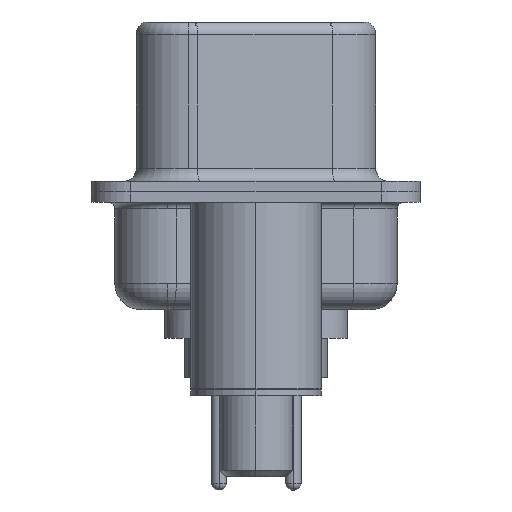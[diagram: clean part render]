
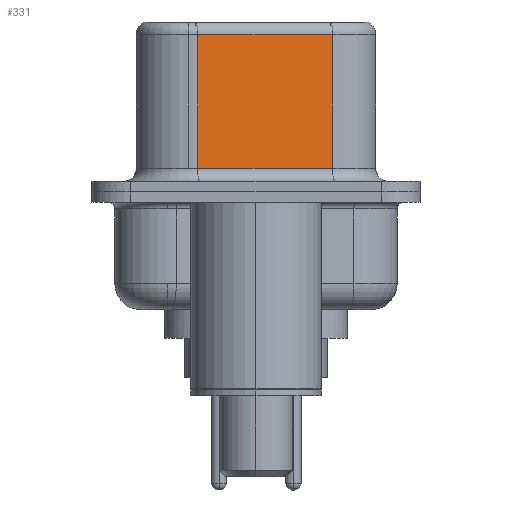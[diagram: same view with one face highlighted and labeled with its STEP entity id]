
A CAD part, left-side view. The second image highlights one B-rep face of the part: STEP entity #331.
In plain terms, the highlighted planar face has unit normal (-0.985, -0.174, 0).
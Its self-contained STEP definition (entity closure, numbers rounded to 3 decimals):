
#331 = ADVANCED_FACE ( 'NONE', ( #4750 ), #9313, .F. ) ;
#768 = ORIENTED_EDGE ( 'NONE', *, *, #12194, .T. ) ;
#1760 = DIRECTION ( 'NONE',  ( 0.174, -0.985, 0. ) ) ;
#2746 = CARTESIAN_POINT ( 'NONE',  ( 3.67, 2.233, 6.52 ) ) ;
#3579 = LINE ( 'NONE', #2746, #11378 ) ;
#4750 = FACE_OUTER_BOUND ( 'NONE', #9979, .T. ) ;
#4772 = ORIENTED_EDGE ( 'NONE', *, *, #19512, .T. ) ;
#5371 = VECTOR ( 'NONE', #1760, 1000. ) ;
#5804 = ORIENTED_EDGE ( 'NONE', *, *, #12025, .F. ) ;
#6564 = VECTOR ( 'NONE', #10188, 1000. ) ;
#6974 = DIRECTION ( 'NONE',  ( 0.985, 0.174, 0. ) ) ;
#7057 = CARTESIAN_POINT ( 'NONE',  ( 4.58, -2.927, 6.52 ) ) ;
#7122 = VERTEX_POINT ( 'NONE', #19516 ) ;
#7389 = CARTESIAN_POINT ( 'NONE',  ( 4.58, -2.927, 6.02 ) ) ;
#8090 = DIRECTION ( 'NONE',  ( -0.174, 0.985, 0. ) ) ;
#9108 = CARTESIAN_POINT ( 'NONE',  ( 4.58, -2.927, 6.52 ) ) ;
#9313 = PLANE ( 'NONE',  #11503 ) ;
#9979 = EDGE_LOOP ( 'NONE', ( #5804, #4772, #768, #16064 ) ) ;
#10025 = EDGE_CURVE ( 'NONE', #11095, #11278, #17002, .T. ) ;
#10188 = DIRECTION ( 'NONE',  ( 0., 0., -1. ) ) ;
#10575 = DIRECTION ( 'NONE',  ( 0., 0., -1. ) ) ;
#10680 = LINE ( 'NONE', #7057, #6564 ) ;
#10826 = CARTESIAN_POINT ( 'NONE',  ( 4.58, -2.927, 0.9 ) ) ;
#10930 = VECTOR ( 'NONE', #14954, 1000. ) ;
#11095 = VERTEX_POINT ( 'NONE', #14836 ) ;
#11278 = VERTEX_POINT ( 'NONE', #10826 ) ;
#11378 = VECTOR ( 'NONE', #10575, 1000. ) ;
#11503 = AXIS2_PLACEMENT_3D ( 'NONE', #9108, #6974, #8090 ) ;
#12025 = EDGE_CURVE ( 'NONE', #16103, #11278, #10680, .T. ) ;
#12194 = EDGE_CURVE ( 'NONE', #7122, #11095, #3579, .T. ) ;
#12607 = CARTESIAN_POINT ( 'NONE',  ( 4.58, -2.927, 0.9 ) ) ;
#14836 = CARTESIAN_POINT ( 'NONE',  ( 3.67, 2.233, 0.9 ) ) ;
#14954 = DIRECTION ( 'NONE',  ( -0.174, 0.985, 0. ) ) ;
#15226 = CARTESIAN_POINT ( 'NONE',  ( 4.58, -2.927, 6.02 ) ) ;
#16064 = ORIENTED_EDGE ( 'NONE', *, *, #10025, .T. ) ;
#16103 = VERTEX_POINT ( 'NONE', #15226 ) ;
#17002 = LINE ( 'NONE', #12607, #5371 ) ;
#19512 = EDGE_CURVE ( 'NONE', #16103, #7122, #19837, .T. ) ;
#19516 = CARTESIAN_POINT ( 'NONE',  ( 3.67, 2.233, 6.02 ) ) ;
#19837 = LINE ( 'NONE', #7389, #10930 ) ;
